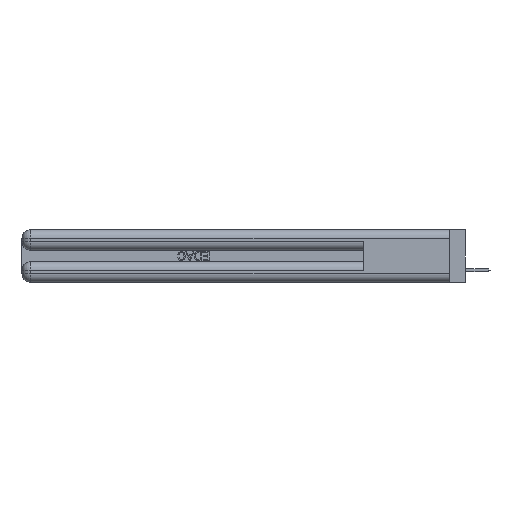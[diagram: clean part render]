
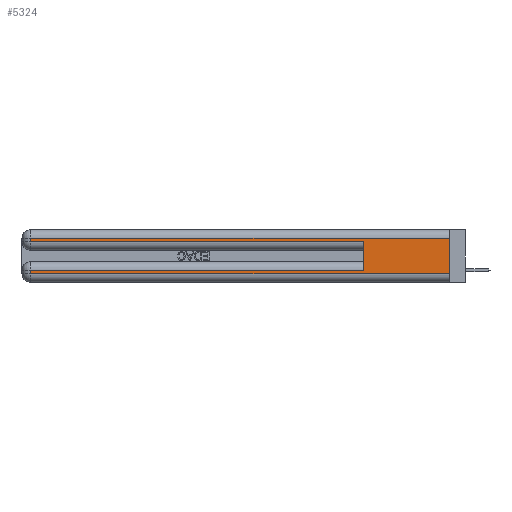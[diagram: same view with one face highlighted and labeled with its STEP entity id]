
A CAD part, left-side view. The second image highlights one B-rep face of the part: STEP entity #5324.
In plain terms, the highlighted planar face has unit normal (-1, 0, 0).
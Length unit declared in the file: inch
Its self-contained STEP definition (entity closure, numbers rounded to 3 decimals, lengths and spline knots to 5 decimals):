
#137 = VECTOR ( 'NONE', #44832, 39.37008 ) ;
#1260 = DIRECTION ( 'NONE',  ( 0., 0., -1. ) ) ;
#1476 = DIRECTION ( 'NONE',  ( 0., 1., 0. ) ) ;
#1769 = VERTEX_POINT ( 'NONE', #45468 ) ;
#1913 = CARTESIAN_POINT ( 'NONE',  ( 0., 2.94, 0.31 ) ) ;
#2534 = EDGE_CURVE ( 'NONE', #52338, #35474, #7131, .T. ) ;
#2807 = EDGE_CURVE ( 'NONE', #9056, #36328, #31588, .T. ) ;
#3058 = CARTESIAN_POINT ( 'NONE',  ( 0., 0.6, 0.145 ) ) ;
#3128 = VECTOR ( 'NONE', #1476, 39.37008 ) ;
#3457 = ORIENTED_EDGE ( 'NONE', *, *, #21691, .F. ) ;
#4074 = CARTESIAN_POINT ( 'NONE',  ( 0., 0., 0.06 ) ) ;
#5324 = ADVANCED_FACE ( 'NONE', ( #33322 ), #13901, .F. ) ;
#7131 = LINE ( 'NONE', #30944, #3128 ) ;
#7651 = EDGE_CURVE ( 'NONE', #36328, #1769, #40947, .T. ) ;
#8049 = VERTEX_POINT ( 'NONE', #52657 ) ;
#8620 = VECTOR ( 'NONE', #47335, 39.37008 ) ;
#9056 = VERTEX_POINT ( 'NONE', #39869 ) ;
#10167 = CARTESIAN_POINT ( 'NONE',  ( 0., 0., 0.06 ) ) ;
#11585 = CARTESIAN_POINT ( 'NONE',  ( 0., 2.94, 0.37 ) ) ;
#12603 = LINE ( 'NONE', #17970, #8620 ) ;
#12625 = DIRECTION ( 'NONE',  ( 0., -1., 0. ) ) ;
#12745 = LINE ( 'NONE', #3058, #137 ) ;
#13901 = PLANE ( 'NONE',  #38600 ) ;
#14274 = DIRECTION ( 'NONE',  ( 0., -1., 0. ) ) ;
#16662 = LINE ( 'NONE', #37530, #31147 ) ;
#17812 = DIRECTION ( 'NONE',  ( 1., 0., 0. ) ) ;
#17970 = CARTESIAN_POINT ( 'NONE',  ( 0., 0., 0.37 ) ) ;
#18847 = ORIENTED_EDGE ( 'NONE', *, *, #2807, .T. ) ;
#20795 = LINE ( 'NONE', #10167, #24131 ) ;
#20798 = CARTESIAN_POINT ( 'NONE',  ( 0., 2.94, 0.37 ) ) ;
#21691 = EDGE_CURVE ( 'NONE', #52338, #24108, #12603, .T. ) ;
#21861 = DIRECTION ( 'NONE',  ( 0., 0., -1. ) ) ;
#22252 = CARTESIAN_POINT ( 'NONE',  ( 0., 0., 0.37 ) ) ;
#24108 = VERTEX_POINT ( 'NONE', #4074 ) ;
#24131 = VECTOR ( 'NONE', #14274, 39.37008 ) ;
#24351 = EDGE_CURVE ( 'NONE', #35474, #25966, #44297, .T. ) ;
#24850 = ORIENTED_EDGE ( 'NONE', *, *, #37695, .F. ) ;
#25860 = DIRECTION ( 'NONE',  ( 0., 1., 0. ) ) ;
#25966 = VERTEX_POINT ( 'NONE', #43834 ) ;
#28880 = CARTESIAN_POINT ( 'NONE',  ( 0., 0., 0.085 ) ) ;
#30446 = ORIENTED_EDGE ( 'NONE', *, *, #2534, .T. ) ;
#30944 = CARTESIAN_POINT ( 'NONE',  ( 0., 0., 0.31 ) ) ;
#31147 = VECTOR ( 'NONE', #12625, 39.37008 ) ;
#31543 = ORIENTED_EDGE ( 'NONE', *, *, #24351, .T. ) ;
#31588 = LINE ( 'NONE', #28880, #48915 ) ;
#32563 = DIRECTION ( 'NONE',  ( 0., 0., -1. ) ) ;
#33322 = FACE_OUTER_BOUND ( 'NONE', #54162, .T. ) ;
#34396 = ORIENTED_EDGE ( 'NONE', *, *, #7651, .T. ) ;
#35474 = VERTEX_POINT ( 'NONE', #1913 ) ;
#35733 = EDGE_CURVE ( 'NONE', #25966, #8049, #16662, .T. ) ;
#36328 = VERTEX_POINT ( 'NONE', #54906 ) ;
#37530 = CARTESIAN_POINT ( 'NONE',  ( 0., 0., 0.285 ) ) ;
#37695 = EDGE_CURVE ( 'NONE', #9056, #8049, #12745, .T. ) ;
#38600 = AXIS2_PLACEMENT_3D ( 'NONE', #22252, #17812, #1260 ) ;
#39869 = CARTESIAN_POINT ( 'NONE',  ( 0., 0.6, 0.085 ) ) ;
#40836 = CARTESIAN_POINT ( 'NONE',  ( 0., 0., 0.31 ) ) ;
#40947 = LINE ( 'NONE', #20798, #47576 ) ;
#41466 = ORIENTED_EDGE ( 'NONE', *, *, #35733, .T. ) ;
#43834 = CARTESIAN_POINT ( 'NONE',  ( 0., 2.94, 0.285 ) ) ;
#44297 = LINE ( 'NONE', #11585, #50292 ) ;
#44827 = EDGE_CURVE ( 'NONE', #1769, #24108, #20795, .T. ) ;
#44832 = DIRECTION ( 'NONE',  ( 0., 0., 1. ) ) ;
#45468 = CARTESIAN_POINT ( 'NONE',  ( 0., 2.94, 0.06 ) ) ;
#46849 = ORIENTED_EDGE ( 'NONE', *, *, #44827, .T. ) ;
#47335 = DIRECTION ( 'NONE',  ( 0., 0., -1. ) ) ;
#47576 = VECTOR ( 'NONE', #21861, 39.37008 ) ;
#48915 = VECTOR ( 'NONE', #25860, 39.37008 ) ;
#50292 = VECTOR ( 'NONE', #32563, 39.37008 ) ;
#52338 = VERTEX_POINT ( 'NONE', #40836 ) ;
#52657 = CARTESIAN_POINT ( 'NONE',  ( 0., 0.6, 0.285 ) ) ;
#54162 = EDGE_LOOP ( 'NONE', ( #3457, #30446, #31543, #41466, #24850, #18847, #34396, #46849 ) ) ;
#54906 = CARTESIAN_POINT ( 'NONE',  ( 0., 2.94, 0.085 ) ) ;
